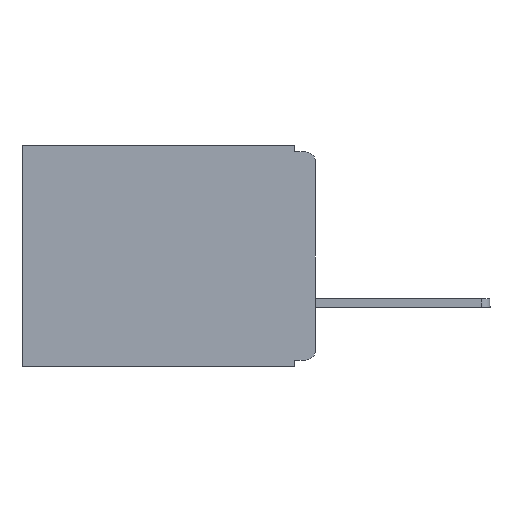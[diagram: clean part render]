
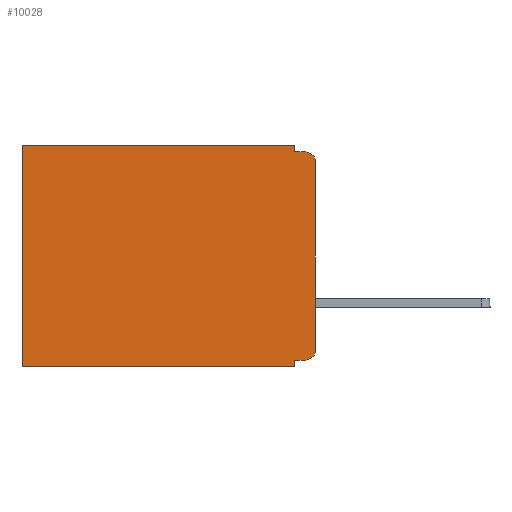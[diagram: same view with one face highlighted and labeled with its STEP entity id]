
A CAD part, left-side view. The second image highlights one B-rep face of the part: STEP entity #10028.
In plain terms, the highlighted planar face has unit normal (-1, 0, 0).
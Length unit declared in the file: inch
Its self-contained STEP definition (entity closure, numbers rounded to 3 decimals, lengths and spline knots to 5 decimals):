
#51 = LINE ( 'NONE', #8139, #5209 ) ;
#75 = VERTEX_POINT ( 'NONE', #5928 ) ;
#206 = DIRECTION ( 'NONE',  ( 0., 0., -1. ) ) ;
#351 = AXIS2_PLACEMENT_3D ( 'NONE', #6369, #4211, #12033 ) ;
#409 = VERTEX_POINT ( 'NONE', #12413 ) ;
#701 = AXIS2_PLACEMENT_3D ( 'NONE', #9164, #11525, #206 ) ;
#824 = VERTEX_POINT ( 'NONE', #2549 ) ;
#868 = CARTESIAN_POINT ( 'NONE',  ( 0.3, 0., -0.025 ) ) ;
#1612 = CARTESIAN_POINT ( 'NONE',  ( 0.3, 0.437, -0.33 ) ) ;
#1831 = LINE ( 'NONE', #3964, #7452 ) ;
#2026 = DIRECTION ( 'NONE',  ( 0., 1., 0. ) ) ;
#2275 = VECTOR ( 'NONE', #4898, 39.37008 ) ;
#2277 = VERTEX_POINT ( 'NONE', #868 ) ;
#2539 = ORIENTED_EDGE ( 'NONE', *, *, #6545, .F. ) ;
#2549 = CARTESIAN_POINT ( 'NONE',  ( 0.3, 0.031, -0.32 ) ) ;
#2904 = ORIENTED_EDGE ( 'NONE', *, *, #4022, .F. ) ;
#3072 = CIRCLE ( 'NONE', #351, 0.015 ) ;
#3092 = CARTESIAN_POINT ( 'NONE',  ( 0.3, 0., 0. ) ) ;
#3177 = CARTESIAN_POINT ( 'NONE',  ( 0.3, 0.031, 0. ) ) ;
#3547 = CARTESIAN_POINT ( 'NONE',  ( 0.3, 0., -0.33 ) ) ;
#3602 = VECTOR ( 'NONE', #10427, 39.37008 ) ;
#3664 = EDGE_CURVE ( 'NONE', #2277, #10291, #7891, .T. ) ;
#3753 = LINE ( 'NONE', #3092, #6139 ) ;
#3896 = ORIENTED_EDGE ( 'NONE', *, *, #7397, .F. ) ;
#3964 = CARTESIAN_POINT ( 'NONE',  ( 0.3, 0.031, -0.33 ) ) ;
#4022 = EDGE_CURVE ( 'NONE', #12490, #6059, #8485, .T. ) ;
#4207 = LINE ( 'NONE', #3177, #9000 ) ;
#4211 = DIRECTION ( 'NONE',  ( -1., 0., 0. ) ) ;
#4421 = EDGE_CURVE ( 'NONE', #75, #824, #11335, .T. ) ;
#4518 = EDGE_CURVE ( 'NONE', #2277, #6059, #12388, .T. ) ;
#4590 = DIRECTION ( 'NONE',  ( 0., 0., -1. ) ) ;
#4708 = EDGE_CURVE ( 'NONE', #75, #10291, #3072, .T. ) ;
#4892 = CARTESIAN_POINT ( 'NONE',  ( 0.3, 0.015, -0.01 ) ) ;
#4898 = DIRECTION ( 'NONE',  ( 0., 0., -1. ) ) ;
#4988 = DIRECTION ( 'NONE',  ( 0., 0., -1. ) ) ;
#5066 = DIRECTION ( 'NONE',  ( 0., 0., -1. ) ) ;
#5209 = VECTOR ( 'NONE', #5066, 39.37008 ) ;
#5371 = ORIENTED_EDGE ( 'NONE', *, *, #5897, .T. ) ;
#5527 = FACE_OUTER_BOUND ( 'NONE', #8411, .T. ) ;
#5697 = VECTOR ( 'NONE', #10030, 39.37008 ) ;
#5844 = ORIENTED_EDGE ( 'NONE', *, *, #4708, .T. ) ;
#5897 = EDGE_CURVE ( 'NONE', #10494, #6460, #51, .T. ) ;
#5928 = CARTESIAN_POINT ( 'NONE',  ( 0.3, 0.015, -0.32 ) ) ;
#6059 = VERTEX_POINT ( 'NONE', #4892 ) ;
#6067 = AXIS2_PLACEMENT_3D ( 'NONE', #3547, #10463, #4590 ) ;
#6139 = VECTOR ( 'NONE', #2026, 39.37008 ) ;
#6369 = CARTESIAN_POINT ( 'NONE',  ( 0.3, 0.015, -0.305 ) ) ;
#6460 = VERTEX_POINT ( 'NONE', #1612 ) ;
#6493 = CARTESIAN_POINT ( 'NONE',  ( 0.3, 0.437, 0. ) ) ;
#6545 = EDGE_CURVE ( 'NONE', #10121, #6460, #11783, .T. ) ;
#6604 = PLANE ( 'NONE',  #6067 ) ;
#6997 = CARTESIAN_POINT ( 'NONE',  ( 0.3, 0.031, -0.01 ) ) ;
#7115 = EDGE_CURVE ( 'NONE', #409, #12490, #4207, .T. ) ;
#7317 = VECTOR ( 'NONE', #9296, 39.37008 ) ;
#7397 = EDGE_CURVE ( 'NONE', #824, #10121, #1831, .T. ) ;
#7452 = VECTOR ( 'NONE', #4988, 39.37008 ) ;
#7891 = LINE ( 'NONE', #11726, #2275 ) ;
#7893 = CARTESIAN_POINT ( 'NONE',  ( 0.3, 0.031, -0.33 ) ) ;
#8139 = CARTESIAN_POINT ( 'NONE',  ( 0.3, 0.437, -0.33 ) ) ;
#8149 = ORIENTED_EDGE ( 'NONE', *, *, #4421, .F. ) ;
#8239 = ORIENTED_EDGE ( 'NONE', *, *, #3664, .F. ) ;
#8411 = EDGE_LOOP ( 'NONE', ( #8239, #8520, #2904, #9159, #10400, #5371, #2539, #3896, #8149, #5844 ) ) ;
#8485 = LINE ( 'NONE', #12249, #5697 ) ;
#8520 = ORIENTED_EDGE ( 'NONE', *, *, #4518, .T. ) ;
#9000 = VECTOR ( 'NONE', #11118, 39.37008 ) ;
#9159 = ORIENTED_EDGE ( 'NONE', *, *, #7115, .F. ) ;
#9164 = CARTESIAN_POINT ( 'NONE',  ( 0.3, 0.015, -0.025 ) ) ;
#9296 = DIRECTION ( 'NONE',  ( 0., 1., 0. ) ) ;
#9327 = CARTESIAN_POINT ( 'NONE',  ( 0.3, 0., -0.33 ) ) ;
#10028 = ADVANCED_FACE ( 'NONE', ( #5527 ), #6604, .F. ) ;
#10030 = DIRECTION ( 'NONE',  ( 0., -1., 0. ) ) ;
#10032 = CARTESIAN_POINT ( 'NONE',  ( 0.3, 0., -0.305 ) ) ;
#10121 = VERTEX_POINT ( 'NONE', #7893 ) ;
#10291 = VERTEX_POINT ( 'NONE', #10032 ) ;
#10344 = EDGE_CURVE ( 'NONE', #409, #10494, #3753, .T. ) ;
#10400 = ORIENTED_EDGE ( 'NONE', *, *, #10344, .T. ) ;
#10427 = DIRECTION ( 'NONE',  ( 0., 1., 0. ) ) ;
#10463 = DIRECTION ( 'NONE',  ( 1., 0., 0. ) ) ;
#10494 = VERTEX_POINT ( 'NONE', #6493 ) ;
#11118 = DIRECTION ( 'NONE',  ( 0., 0., -1. ) ) ;
#11335 = LINE ( 'NONE', #11834, #3602 ) ;
#11525 = DIRECTION ( 'NONE',  ( -1., 0., 0. ) ) ;
#11726 = CARTESIAN_POINT ( 'NONE',  ( 0.3, 0., -0.33 ) ) ;
#11783 = LINE ( 'NONE', #9327, #7317 ) ;
#11834 = CARTESIAN_POINT ( 'NONE',  ( 0.3, 0., -0.32 ) ) ;
#12033 = DIRECTION ( 'NONE',  ( 0., 0., -1. ) ) ;
#12249 = CARTESIAN_POINT ( 'NONE',  ( 0.3, 0., -0.01 ) ) ;
#12388 = CIRCLE ( 'NONE', #701, 0.015 ) ;
#12413 = CARTESIAN_POINT ( 'NONE',  ( 0.3, 0.031, 0. ) ) ;
#12490 = VERTEX_POINT ( 'NONE', #6997 ) ;
